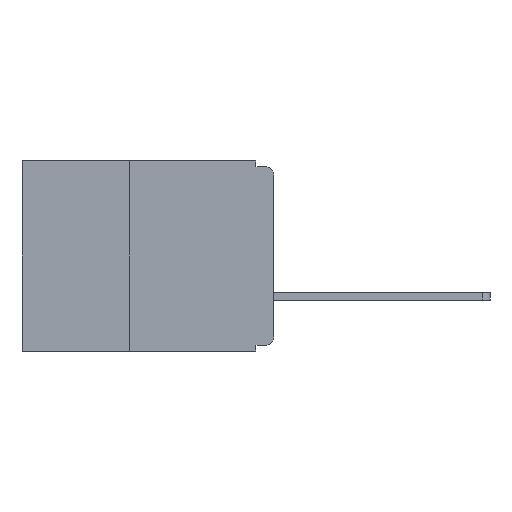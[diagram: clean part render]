
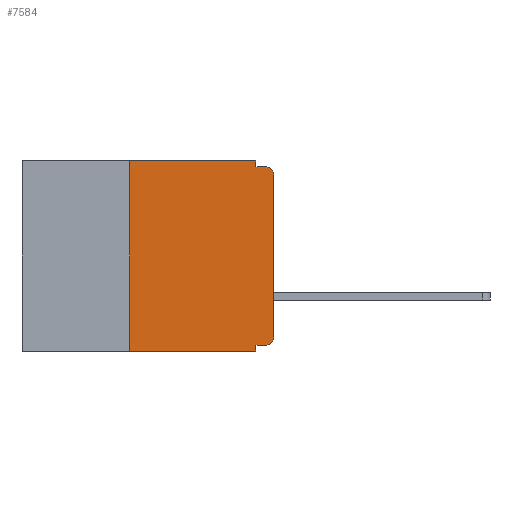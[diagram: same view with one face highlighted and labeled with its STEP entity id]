
A CAD part, left-side view. The second image highlights one B-rep face of the part: STEP entity #7584.
In plain terms, the highlighted planar face has unit normal (-1, 0, 0).
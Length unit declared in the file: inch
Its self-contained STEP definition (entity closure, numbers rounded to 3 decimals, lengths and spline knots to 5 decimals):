
#447 = FACE_OUTER_BOUND ( 'NONE', #5887, .T. ) ;
#560 = EDGE_CURVE ( 'NONE', #10105, #14305, #1891, .T. ) ;
#703 = EDGE_CURVE ( 'NONE', #5691, #14305, #1216, .T. ) ;
#732 = EDGE_CURVE ( 'NONE', #5691, #1603, #1261, .T. ) ;
#937 = EDGE_CURVE ( 'NONE', #14148, #11558, #11158, .T. ) ;
#949 = VECTOR ( 'NONE', #19151, 39.37008 ) ;
#1006 = VECTOR ( 'NONE', #6211, 39.37008 ) ;
#1035 = VECTOR ( 'NONE', #14517, 39.37008 ) ;
#1077 = LINE ( 'NONE', #9068, #1035 ) ;
#1199 = VECTOR ( 'NONE', #18717, 39.37008 ) ;
#1207 = DIRECTION ( 'NONE',  ( 0., 0., -1. ) ) ;
#1216 = LINE ( 'NONE', #2801, #1199 ) ;
#1261 = LINE ( 'NONE', #16470, #949 ) ;
#1375 = LINE ( 'NONE', #6479, #1006 ) ;
#1603 = VERTEX_POINT ( 'NONE', #17781 ) ;
#1644 = EDGE_CURVE ( 'NONE', #11558, #5453, #1077, .T. ) ;
#1868 = VECTOR ( 'NONE', #19105, 39.37008 ) ;
#1891 = LINE ( 'NONE', #16925, #1868 ) ;
#2208 = CARTESIAN_POINT ( 'NONE',  ( 0., 0.031, -0.01 ) ) ;
#2265 = EDGE_CURVE ( 'NONE', #11864, #14574, #16825, .T. ) ;
#2373 = AXIS2_PLACEMENT_3D ( 'NONE', #4345, #2490, #1207 ) ;
#2490 = DIRECTION ( 'NONE',  ( 1., 0., 0. ) ) ;
#2801 = CARTESIAN_POINT ( 'NONE',  ( 0., 0.437, -0.33 ) ) ;
#2867 = VERTEX_POINT ( 'NONE', #6356 ) ;
#3434 = CARTESIAN_POINT ( 'NONE',  ( 0., 0., -0.025 ) ) ;
#3708 = PLANE ( 'NONE',  #2373 ) ;
#4143 = CARTESIAN_POINT ( 'NONE',  ( 0., 0.031, 0. ) ) ;
#4345 = CARTESIAN_POINT ( 'NONE',  ( 0., 0.437, 0. ) ) ;
#4652 = CARTESIAN_POINT ( 'NONE',  ( 0., 0.031, 0. ) ) ;
#5453 = VERTEX_POINT ( 'NONE', #13307 ) ;
#5691 = VERTEX_POINT ( 'NONE', #9032 ) ;
#5887 = EDGE_LOOP ( 'NONE', ( #10119, #10805, #10946, #11366, #11496, #11523, #11996, #12037, #12202, #12362 ) ) ;
#6211 = DIRECTION ( 'NONE',  ( 0., -1., 0. ) ) ;
#6356 = CARTESIAN_POINT ( 'NONE',  ( 0., 0.015, -0.32 ) ) ;
#6479 = CARTESIAN_POINT ( 'NONE',  ( 0., 0.437, 0. ) ) ;
#7584 = ADVANCED_FACE ( 'NONE', ( #447 ), #3708, .F. ) ;
#9032 = CARTESIAN_POINT ( 'NONE',  ( 0., 0.25, -0.33 ) ) ;
#9068 = CARTESIAN_POINT ( 'NONE',  ( 0., 0., -0.01 ) ) ;
#10015 = VECTOR ( 'NONE', #16026, 39.37008 ) ;
#10103 = LINE ( 'NONE', #16060, #10015 ) ;
#10105 = VERTEX_POINT ( 'NONE', #17504 ) ;
#10119 = ORIENTED_EDGE ( 'NONE', *, *, #2265, .T. ) ;
#10603 = DIRECTION ( 'NONE',  ( 0., 0., 1. ) ) ;
#10805 = ORIENTED_EDGE ( 'NONE', *, *, #18473, .T. ) ;
#10946 = ORIENTED_EDGE ( 'NONE', *, *, #1644, .F. ) ;
#11093 = CIRCLE ( 'NONE', #18869, 0.015 ) ;
#11158 = LINE ( 'NONE', #4143, #11759 ) ;
#11366 = ORIENTED_EDGE ( 'NONE', *, *, #937, .F. ) ;
#11401 = CARTESIAN_POINT ( 'NONE',  ( 0., 0., -0.305 ) ) ;
#11496 = ORIENTED_EDGE ( 'NONE', *, *, #17370, .F. ) ;
#11521 = CIRCLE ( 'NONE', #12956, 0.015 ) ;
#11523 = ORIENTED_EDGE ( 'NONE', *, *, #732, .F. ) ;
#11558 = VERTEX_POINT ( 'NONE', #2208 ) ;
#11759 = VECTOR ( 'NONE', #13344, 39.37008 ) ;
#11864 = VERTEX_POINT ( 'NONE', #11401 ) ;
#11996 = ORIENTED_EDGE ( 'NONE', *, *, #703, .T. ) ;
#12037 = ORIENTED_EDGE ( 'NONE', *, *, #560, .F. ) ;
#12202 = ORIENTED_EDGE ( 'NONE', *, *, #18595, .F. ) ;
#12362 = ORIENTED_EDGE ( 'NONE', *, *, #18423, .T. ) ;
#12956 = AXIS2_PLACEMENT_3D ( 'NONE', #19080, #19036, #19022 ) ;
#13307 = CARTESIAN_POINT ( 'NONE',  ( 0., 0.015, -0.01 ) ) ;
#13344 = DIRECTION ( 'NONE',  ( 0., 0., -1. ) ) ;
#14148 = VERTEX_POINT ( 'NONE', #4652 ) ;
#14305 = VERTEX_POINT ( 'NONE', #16343 ) ;
#14517 = DIRECTION ( 'NONE',  ( 0., -1., 0. ) ) ;
#14574 = VERTEX_POINT ( 'NONE', #3434 ) ;
#16026 = DIRECTION ( 'NONE',  ( 0., 1., 0. ) ) ;
#16060 = CARTESIAN_POINT ( 'NONE',  ( 0., 0., -0.32 ) ) ;
#16343 = CARTESIAN_POINT ( 'NONE',  ( 0., 0.031, -0.33 ) ) ;
#16470 = CARTESIAN_POINT ( 'NONE',  ( 0., 0.25, -0.33 ) ) ;
#16808 = VECTOR ( 'NONE', #10603, 39.37008 ) ;
#16825 = LINE ( 'NONE', #17664, #16808 ) ;
#16925 = CARTESIAN_POINT ( 'NONE',  ( 0., 0.031, -0.33 ) ) ;
#17370 = EDGE_CURVE ( 'NONE', #1603, #14148, #1375, .T. ) ;
#17504 = CARTESIAN_POINT ( 'NONE',  ( 0., 0.031, -0.32 ) ) ;
#17664 = CARTESIAN_POINT ( 'NONE',  ( 0., 0., 0. ) ) ;
#17781 = CARTESIAN_POINT ( 'NONE',  ( 0., 0.25, 0. ) ) ;
#18038 = DIRECTION ( 'NONE',  ( 0., 0., -1. ) ) ;
#18079 = DIRECTION ( 'NONE',  ( -1., 0., 0. ) ) ;
#18120 = CARTESIAN_POINT ( 'NONE',  ( 0., 0.015, -0.025 ) ) ;
#18423 = EDGE_CURVE ( 'NONE', #2867, #11864, #11521, .T. ) ;
#18473 = EDGE_CURVE ( 'NONE', #14574, #5453, #11093, .T. ) ;
#18595 = EDGE_CURVE ( 'NONE', #2867, #10105, #10103, .T. ) ;
#18717 = DIRECTION ( 'NONE',  ( 0., -1., 0. ) ) ;
#18869 = AXIS2_PLACEMENT_3D ( 'NONE', #18120, #18079, #18038 ) ;
#19022 = DIRECTION ( 'NONE',  ( 0., 0., -1. ) ) ;
#19036 = DIRECTION ( 'NONE',  ( -1., 0., 0. ) ) ;
#19080 = CARTESIAN_POINT ( 'NONE',  ( 0., 0.015, -0.305 ) ) ;
#19105 = DIRECTION ( 'NONE',  ( 0., 0., -1. ) ) ;
#19151 = DIRECTION ( 'NONE',  ( 0., 0., 1. ) ) ;
